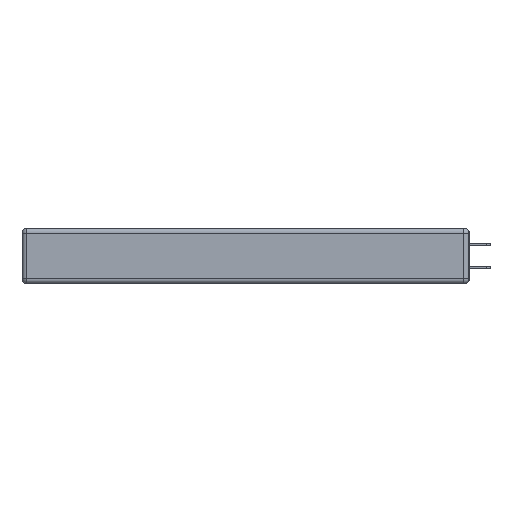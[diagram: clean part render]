
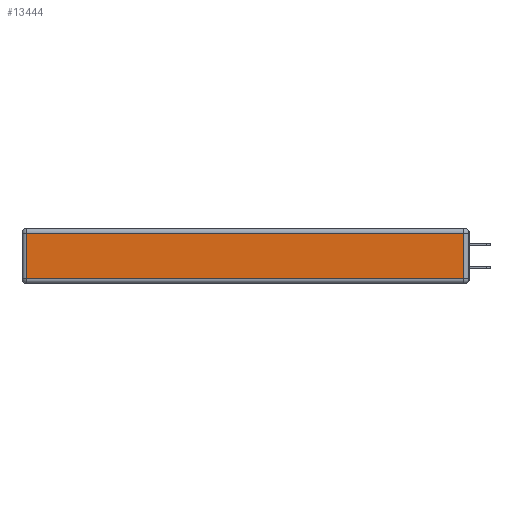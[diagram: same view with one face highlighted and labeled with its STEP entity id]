
A CAD part, left-side view. The second image highlights one B-rep face of the part: STEP entity #13444.
In plain terms, the highlighted planar face has unit normal (-1, 0, 0).
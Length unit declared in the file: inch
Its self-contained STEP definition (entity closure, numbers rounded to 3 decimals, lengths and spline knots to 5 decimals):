
#101 = DIRECTION ( 'NONE',  ( 0., 0., -1. ) ) ;
#156 = AXIS2_PLACEMENT_3D ( 'NONE', #5460, #15642, #5537 ) ;
#239 = EDGE_LOOP ( 'NONE', ( #4194, #6414, #7011, #21268 ) ) ;
#654 = EDGE_CURVE ( 'NONE', #20374, #4253, #6331, .T. ) ;
#1678 = VECTOR ( 'NONE', #101, 39.37008 ) ;
#1847 = EDGE_CURVE ( 'NONE', #13672, #2479, #4562, .T. ) ;
#2479 = VERTEX_POINT ( 'NONE', #20860 ) ;
#3577 = PLANE ( 'NONE',  #156 ) ;
#3644 = CARTESIAN_POINT ( 'NONE',  ( 0., 0.03, -0.03 ) ) ;
#3896 = DIRECTION ( 'NONE',  ( 0., -1., 0. ) ) ;
#3993 = CARTESIAN_POINT ( 'NONE',  ( 0., 2.75, -0.03 ) ) ;
#4182 = VECTOR ( 'NONE', #7362, 39.37008 ) ;
#4194 = ORIENTED_EDGE ( 'NONE', *, *, #1847, .T. ) ;
#4253 = VERTEX_POINT ( 'NONE', #11389 ) ;
#4562 = LINE ( 'NONE', #9043, #17689 ) ;
#5460 = CARTESIAN_POINT ( 'NONE',  ( 0., 0., -0.343 ) ) ;
#5537 = DIRECTION ( 'NONE',  ( 0., 0., 1. ) ) ;
#6331 = LINE ( 'NONE', #3993, #19461 ) ;
#6414 = ORIENTED_EDGE ( 'NONE', *, *, #7269, .T. ) ;
#7011 = ORIENTED_EDGE ( 'NONE', *, *, #654, .T. ) ;
#7269 = EDGE_CURVE ( 'NONE', #2479, #20374, #17302, .T. ) ;
#7362 = DIRECTION ( 'NONE',  ( 0., 0., 1. ) ) ;
#8766 = CARTESIAN_POINT ( 'NONE',  ( 0., 0.03, -0.343 ) ) ;
#9043 = CARTESIAN_POINT ( 'NONE',  ( 0., 0., -0.313 ) ) ;
#11389 = CARTESIAN_POINT ( 'NONE',  ( 0., 2.72, -0.03 ) ) ;
#12450 = DIRECTION ( 'NONE',  ( 0., 1., 0. ) ) ;
#13444 = ADVANCED_FACE ( 'NONE', ( #15895 ), #3577, .T. ) ;
#13672 = VERTEX_POINT ( 'NONE', #15128 ) ;
#15128 = CARTESIAN_POINT ( 'NONE',  ( 0., 2.72, -0.313 ) ) ;
#15490 = CARTESIAN_POINT ( 'NONE',  ( 0., 2.72, -0.343 ) ) ;
#15642 = DIRECTION ( 'NONE',  ( -1., 0., 0. ) ) ;
#15895 = FACE_OUTER_BOUND ( 'NONE', #239, .T. ) ;
#16661 = LINE ( 'NONE', #15490, #1678 ) ;
#17302 = LINE ( 'NONE', #8766, #4182 ) ;
#17689 = VECTOR ( 'NONE', #3896, 39.37008 ) ;
#18273 = EDGE_CURVE ( 'NONE', #4253, #13672, #16661, .T. ) ;
#19461 = VECTOR ( 'NONE', #12450, 39.37008 ) ;
#20374 = VERTEX_POINT ( 'NONE', #3644 ) ;
#20860 = CARTESIAN_POINT ( 'NONE',  ( 0., 0.03, -0.313 ) ) ;
#21268 = ORIENTED_EDGE ( 'NONE', *, *, #18273, .T. ) ;
